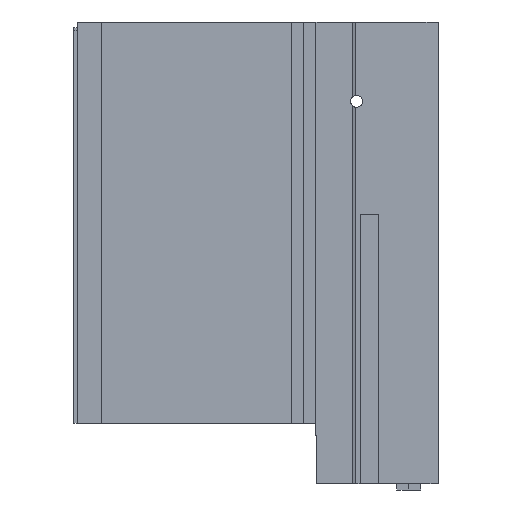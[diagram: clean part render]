
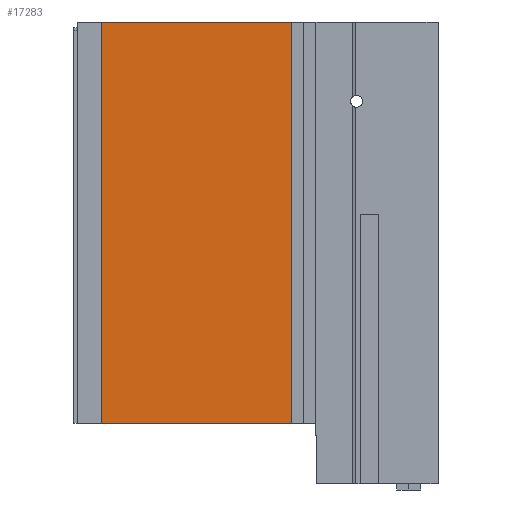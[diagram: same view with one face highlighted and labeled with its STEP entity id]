
A CAD part, left-side view. The second image highlights one B-rep face of the part: STEP entity #17283.
In plain terms, the highlighted planar face has unit normal (-1, 0, 0).
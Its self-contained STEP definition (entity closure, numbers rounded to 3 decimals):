
#8981 = PLANE('',#8982);
#8982 = AXIS2_PLACEMENT_3D('',#8983,#8984,#8985);
#8983 = CARTESIAN_POINT('',(16.25,48.828,76.2));
#8984 = DIRECTION('',(0.,0.,1.));
#8985 = DIRECTION('',(1.,0.,0.));
#14289 = VERTEX_POINT('',#14290);
#14290 = CARTESIAN_POINT('',(-15.,44.828,76.2));
#14304 = PLANE('',#14305);
#14305 = AXIS2_PLACEMENT_3D('',#14306,#14307,#14308);
#14306 = CARTESIAN_POINT('',(-16.364,44.828,76.2));
#14307 = DIRECTION('',(0.,-1.,0.));
#14308 = DIRECTION('',(1.,0.,0.));
#14316 = EDGE_CURVE('',#14289,#14317,#14319,.T.);
#14317 = VERTEX_POINT('',#14318);
#14318 = CARTESIAN_POINT('',(-15.,13.467,76.2));
#14319 = SURFACE_CURVE('',#14320,(#14324,#14331),.PCURVE_S1.);
#14320 = LINE('',#14321,#14322);
#14321 = CARTESIAN_POINT('',(-15.,44.828,76.2));
#14322 = VECTOR('',#14323,1.);
#14323 = DIRECTION('',(0.,-1.,0.));
#14324 = PCURVE('',#8981,#14325);
#14325 = DEFINITIONAL_REPRESENTATION('',(#14326),#14330);
#14326 = LINE('',#14327,#14328);
#14327 = CARTESIAN_POINT('',(-31.25,-4.));
#14328 = VECTOR('',#14329,1.);
#14329 = DIRECTION('',(0.,-1.));
#14330 = ( GEOMETRIC_REPRESENTATION_CONTEXT(2) 
PARAMETRIC_REPRESENTATION_CONTEXT() REPRESENTATION_CONTEXT('2D SPACE',''
  ) );
#14331 = PCURVE('',#14332,#14337);
#14332 = PLANE('',#14333);
#14333 = AXIS2_PLACEMENT_3D('',#14334,#14335,#14336);
#14334 = CARTESIAN_POINT('',(-15.,44.828,76.2));
#14335 = DIRECTION('',(-1.,0.,0.));
#14336 = DIRECTION('',(0.,-1.,0.));
#14337 = DEFINITIONAL_REPRESENTATION('',(#14338),#14342);
#14338 = LINE('',#14339,#14340);
#14339 = CARTESIAN_POINT('',(0.,0.));
#14340 = VECTOR('',#14341,1.);
#14341 = DIRECTION('',(1.,0.));
#14342 = ( GEOMETRIC_REPRESENTATION_CONTEXT(2) 
PARAMETRIC_REPRESENTATION_CONTEXT() REPRESENTATION_CONTEXT('2D SPACE',''
  ) );
#14360 = PLANE('',#14361);
#14361 = AXIS2_PLACEMENT_3D('',#14362,#14363,#14364);
#14362 = CARTESIAN_POINT('',(-15.,13.467,76.2));
#14363 = DIRECTION('',(0.,1.,0.));
#14364 = DIRECTION('',(-1.,0.,0.));
#15906 = PLANE('',#15907);
#15907 = AXIS2_PLACEMENT_3D('',#15908,#15909,#15910);
#15908 = CARTESIAN_POINT('',(16.25,52.085,10.));
#15909 = DIRECTION('',(0.,0.,1.));
#15910 = DIRECTION('',(0.,-1.,0.));
#17196 = VERTEX_POINT('',#17197);
#17197 = CARTESIAN_POINT('',(-15.,44.828,10.));
#17216 = EDGE_CURVE('',#14289,#17196,#17217,.T.);
#17217 = SURFACE_CURVE('',#17218,(#17222,#17229),.PCURVE_S1.);
#17218 = LINE('',#17219,#17220);
#17219 = CARTESIAN_POINT('',(-15.,44.828,76.2));
#17220 = VECTOR('',#17221,1.);
#17221 = DIRECTION('',(0.,0.,-1.));
#17222 = PCURVE('',#14304,#17223);
#17223 = DEFINITIONAL_REPRESENTATION('',(#17224),#17228);
#17224 = LINE('',#17225,#17226);
#17225 = CARTESIAN_POINT('',(1.364,0.));
#17226 = VECTOR('',#17227,1.);
#17227 = DIRECTION('',(0.,-1.));
#17228 = ( GEOMETRIC_REPRESENTATION_CONTEXT(2) 
PARAMETRIC_REPRESENTATION_CONTEXT() REPRESENTATION_CONTEXT('2D SPACE',''
  ) );
#17229 = PCURVE('',#14332,#17230);
#17230 = DEFINITIONAL_REPRESENTATION('',(#17231),#17235);
#17231 = LINE('',#17232,#17233);
#17232 = CARTESIAN_POINT('',(0.,0.));
#17233 = VECTOR('',#17234,1.);
#17234 = DIRECTION('',(0.,-1.));
#17235 = ( GEOMETRIC_REPRESENTATION_CONTEXT(2) 
PARAMETRIC_REPRESENTATION_CONTEXT() REPRESENTATION_CONTEXT('2D SPACE',''
  ) );
#17283 = ADVANCED_FACE('',(#17284),#14332,.T.);
#17284 = FACE_BOUND('',#17285,.T.);
#17285 = EDGE_LOOP('',(#17286,#17307,#17328,#17329));
#17286 = ORIENTED_EDGE('',*,*,#17287,.F.);
#17287 = EDGE_CURVE('',#17288,#17196,#17290,.T.);
#17288 = VERTEX_POINT('',#17289);
#17289 = CARTESIAN_POINT('',(-15.,13.467,10.));
#17290 = SURFACE_CURVE('',#17291,(#17295,#17301),.PCURVE_S1.);
#17291 = LINE('',#17292,#17293);
#17292 = CARTESIAN_POINT('',(-15.,48.456,10.));
#17293 = VECTOR('',#17294,1.);
#17294 = DIRECTION('',(0.,1.,0.));
#17295 = PCURVE('',#14332,#17296);
#17296 = DEFINITIONAL_REPRESENTATION('',(#17297),#17300);
#17297 = B_SPLINE_CURVE_WITH_KNOTS('',1,(#17298,#17299),.UNSPECIFIED.,
  .F.,.F.,(2,2),(-34.989,-3.629),.PIECEWISE_BEZIER_KNOTS.);
#17298 = CARTESIAN_POINT('',(31.361,-66.2));
#17299 = CARTESIAN_POINT('',(0.,-66.2));
#17300 = ( GEOMETRIC_REPRESENTATION_CONTEXT(2) 
PARAMETRIC_REPRESENTATION_CONTEXT() REPRESENTATION_CONTEXT('2D SPACE',''
  ) );
#17301 = PCURVE('',#15906,#17302);
#17302 = DEFINITIONAL_REPRESENTATION('',(#17303),#17306);
#17303 = B_SPLINE_CURVE_WITH_KNOTS('',1,(#17304,#17305),.UNSPECIFIED.,
  .F.,.F.,(2,2),(-34.989,-3.629),.PIECEWISE_BEZIER_KNOTS.);
#17304 = CARTESIAN_POINT('',(38.618,-31.25));
#17305 = CARTESIAN_POINT('',(7.257,-31.25));
#17306 = ( GEOMETRIC_REPRESENTATION_CONTEXT(2) 
PARAMETRIC_REPRESENTATION_CONTEXT() REPRESENTATION_CONTEXT('2D SPACE',''
  ) );
#17307 = ORIENTED_EDGE('',*,*,#17308,.F.);
#17308 = EDGE_CURVE('',#14317,#17288,#17309,.T.);
#17309 = SURFACE_CURVE('',#17310,(#17314,#17321),.PCURVE_S1.);
#17310 = LINE('',#17311,#17312);
#17311 = CARTESIAN_POINT('',(-15.,13.467,76.2));
#17312 = VECTOR('',#17313,1.);
#17313 = DIRECTION('',(0.,0.,-1.));
#17314 = PCURVE('',#14332,#17315);
#17315 = DEFINITIONAL_REPRESENTATION('',(#17316),#17320);
#17316 = LINE('',#17317,#17318);
#17317 = CARTESIAN_POINT('',(31.361,0.));
#17318 = VECTOR('',#17319,1.);
#17319 = DIRECTION('',(0.,-1.));
#17320 = ( GEOMETRIC_REPRESENTATION_CONTEXT(2) 
PARAMETRIC_REPRESENTATION_CONTEXT() REPRESENTATION_CONTEXT('2D SPACE',''
  ) );
#17321 = PCURVE('',#14360,#17322);
#17322 = DEFINITIONAL_REPRESENTATION('',(#17323),#17327);
#17323 = LINE('',#17324,#17325);
#17324 = CARTESIAN_POINT('',(0.,0.));
#17325 = VECTOR('',#17326,1.);
#17326 = DIRECTION('',(0.,-1.));
#17327 = ( GEOMETRIC_REPRESENTATION_CONTEXT(2) 
PARAMETRIC_REPRESENTATION_CONTEXT() REPRESENTATION_CONTEXT('2D SPACE',''
  ) );
#17328 = ORIENTED_EDGE('',*,*,#14316,.F.);
#17329 = ORIENTED_EDGE('',*,*,#17216,.T.);
